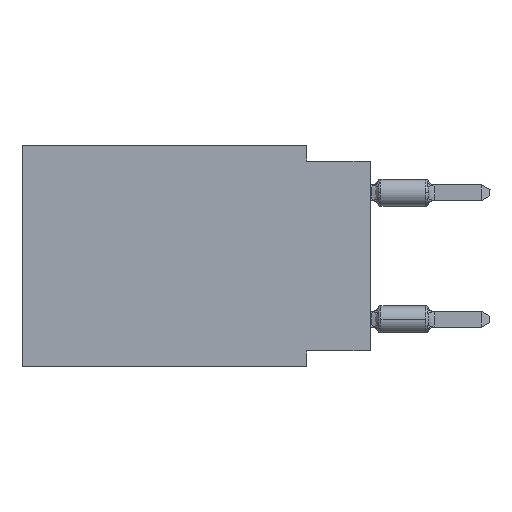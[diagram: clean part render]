
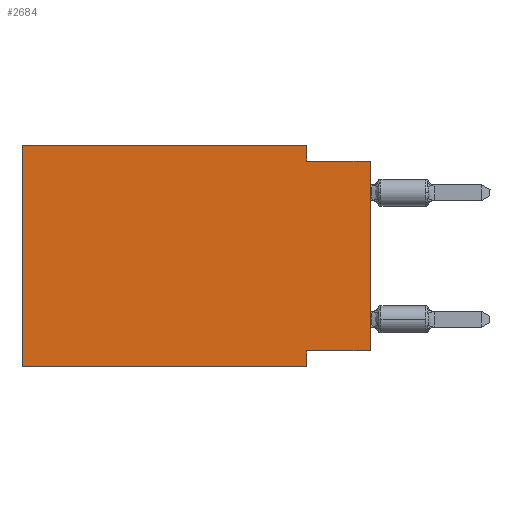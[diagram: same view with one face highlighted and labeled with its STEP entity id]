
A CAD part, left-side view. The second image highlights one B-rep face of the part: STEP entity #2684.
In plain terms, the highlighted planar face has unit normal (-1, 0, 0).
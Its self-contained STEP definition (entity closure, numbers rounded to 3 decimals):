
#1646 = LINE ( 'NONE', #32392, #22734 ) ;
#2210 = FACE_OUTER_BOUND ( 'NONE', #27872, .T. ) ;
#2684 = ADVANCED_FACE ( 'NONE', ( #2210 ), #25389, .F. ) ;
#3534 = DIRECTION ( 'NONE',  ( 0., -1., 0. ) ) ;
#4759 = VERTEX_POINT ( 'NONE', #12415 ) ;
#6854 = VERTEX_POINT ( 'NONE', #8118 ) ;
#8118 = CARTESIAN_POINT ( 'NONE',  ( 0., 13.97, 0. ) ) ;
#8293 = VECTOR ( 'NONE', #34271, 1000. ) ;
#9144 = EDGE_CURVE ( 'NONE', #16366, #15892, #17711, .T. ) ;
#10848 = LINE ( 'NONE', #27659, #23370 ) ;
#11391 = LINE ( 'NONE', #15543, #37479 ) ;
#12062 = CARTESIAN_POINT ( 'NONE',  ( 0., 0., -8.255 ) ) ;
#12415 = CARTESIAN_POINT ( 'NONE',  ( 0., 2.54, -0.635 ) ) ;
#14285 = VERTEX_POINT ( 'NONE', #12062 ) ;
#14337 = VECTOR ( 'NONE', #24147, 1000. ) ;
#14842 = CARTESIAN_POINT ( 'NONE',  ( 0., 13.97, -8.89 ) ) ;
#15155 = CARTESIAN_POINT ( 'NONE',  ( 0., 2.54, 0. ) ) ;
#15543 = CARTESIAN_POINT ( 'NONE',  ( 0., 0., 0. ) ) ;
#15548 = CARTESIAN_POINT ( 'NONE',  ( 0., 0., -0.635 ) ) ;
#15892 = VERTEX_POINT ( 'NONE', #48047 ) ;
#16366 = VERTEX_POINT ( 'NONE', #14842 ) ;
#16818 = EDGE_CURVE ( 'NONE', #14285, #43691, #18394, .T. ) ;
#17460 = DIRECTION ( 'NONE',  ( 0., -1., 0. ) ) ;
#17520 = DIRECTION ( 'NONE',  ( 0., -1., 0. ) ) ;
#17711 = LINE ( 'NONE', #48983, #23175 ) ;
#18038 = EDGE_CURVE ( 'NONE', #42279, #4759, #10848, .T. ) ;
#18394 = LINE ( 'NONE', #18662, #8293 ) ;
#18662 = CARTESIAN_POINT ( 'NONE',  ( 0., 0., -8.255 ) ) ;
#19988 = LINE ( 'NONE', #24662, #14337 ) ;
#20026 = ORIENTED_EDGE ( 'NONE', *, *, #29237, .F. ) ;
#22622 = ORIENTED_EDGE ( 'NONE', *, *, #9144, .T. ) ;
#22734 = VECTOR ( 'NONE', #17520, 1000. ) ;
#23175 = VECTOR ( 'NONE', #17460, 1000. ) ;
#23370 = VECTOR ( 'NONE', #40391, 1000. ) ;
#24147 = DIRECTION ( 'NONE',  ( 0., 0., 1. ) ) ;
#24662 = CARTESIAN_POINT ( 'NONE',  ( 0., 13.97, 0. ) ) ;
#25290 = VERTEX_POINT ( 'NONE', #15548 ) ;
#25389 = PLANE ( 'NONE',  #29484 ) ;
#27472 = LINE ( 'NONE', #40194, #45193 ) ;
#27659 = CARTESIAN_POINT ( 'NONE',  ( 0., 2.54, 0. ) ) ;
#27872 = EDGE_LOOP ( 'NONE', ( #44111, #38053, #40251, #20026, #30388, #22622, #31779, #29445 ) ) ;
#29237 = EDGE_CURVE ( 'NONE', #6854, #42279, #1646, .T. ) ;
#29445 = ORIENTED_EDGE ( 'NONE', *, *, #16818, .F. ) ;
#29484 = AXIS2_PLACEMENT_3D ( 'NONE', #33451, #50128, #38139 ) ;
#30388 = ORIENTED_EDGE ( 'NONE', *, *, #40325, .F. ) ;
#31779 = ORIENTED_EDGE ( 'NONE', *, *, #48004, .F. ) ;
#32392 = CARTESIAN_POINT ( 'NONE',  ( 0., 13.97, 0. ) ) ;
#33451 = CARTESIAN_POINT ( 'NONE',  ( 0., 13.97, 0. ) ) ;
#34271 = DIRECTION ( 'NONE',  ( 0., 1., 0. ) ) ;
#36629 = EDGE_CURVE ( 'NONE', #14285, #25290, #11391, .T. ) ;
#36764 = VECTOR ( 'NONE', #3534, 1000. ) ;
#37479 = VECTOR ( 'NONE', #43145, 1000. ) ;
#38053 = ORIENTED_EDGE ( 'NONE', *, *, #41457, .F. ) ;
#38139 = DIRECTION ( 'NONE',  ( 0., 0., -1. ) ) ;
#38754 = CARTESIAN_POINT ( 'NONE',  ( 0., 2.54, -8.255 ) ) ;
#40194 = CARTESIAN_POINT ( 'NONE',  ( 0., 2.54, -8.89 ) ) ;
#40251 = ORIENTED_EDGE ( 'NONE', *, *, #18038, .F. ) ;
#40325 = EDGE_CURVE ( 'NONE', #16366, #6854, #19988, .T. ) ;
#40391 = DIRECTION ( 'NONE',  ( 0., 0., -1. ) ) ;
#41457 = EDGE_CURVE ( 'NONE', #4759, #25290, #51469, .T. ) ;
#42279 = VERTEX_POINT ( 'NONE', #15155 ) ;
#43145 = DIRECTION ( 'NONE',  ( 0., 0., 1. ) ) ;
#43691 = VERTEX_POINT ( 'NONE', #38754 ) ;
#44111 = ORIENTED_EDGE ( 'NONE', *, *, #36629, .T. ) ;
#44112 = DIRECTION ( 'NONE',  ( 0., 0., -1. ) ) ;
#45193 = VECTOR ( 'NONE', #44112, 1000. ) ;
#48004 = EDGE_CURVE ( 'NONE', #43691, #15892, #27472, .T. ) ;
#48047 = CARTESIAN_POINT ( 'NONE',  ( 0., 2.54, -8.89 ) ) ;
#48983 = CARTESIAN_POINT ( 'NONE',  ( 0., 13.97, -8.89 ) ) ;
#50128 = DIRECTION ( 'NONE',  ( 1., 0., 0. ) ) ;
#51212 = CARTESIAN_POINT ( 'NONE',  ( 0., 0., -0.635 ) ) ;
#51469 = LINE ( 'NONE', #51212, #36764 ) ;
